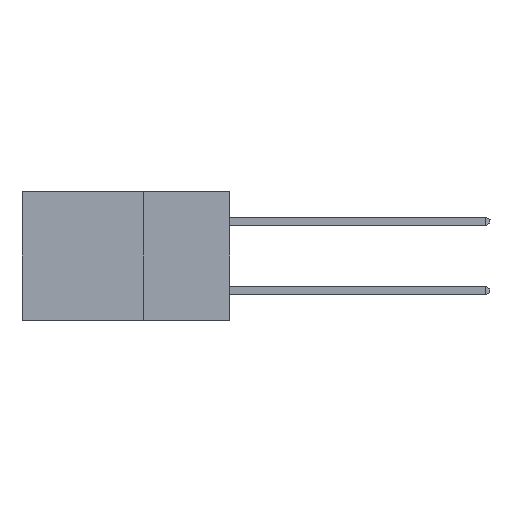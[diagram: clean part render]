
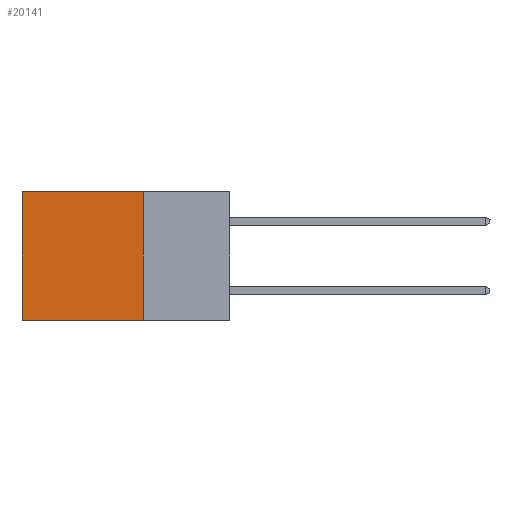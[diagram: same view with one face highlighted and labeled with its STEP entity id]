
A CAD part, left-side view. The second image highlights one B-rep face of the part: STEP entity #20141.
In plain terms, the highlighted planar face has unit normal (-1, 0, 0).
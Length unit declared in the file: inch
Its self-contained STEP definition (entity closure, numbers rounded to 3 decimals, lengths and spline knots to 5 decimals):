
#541 = VERTEX_POINT ( 'NONE', #21755 ) ;
#1035 = DIRECTION ( 'NONE',  ( 0., 0., -1. ) ) ;
#1156 = ORIENTED_EDGE ( 'NONE', *, *, #18524, .T. ) ;
#1758 = ORIENTED_EDGE ( 'NONE', *, *, #5226, .F. ) ;
#1939 = VERTEX_POINT ( 'NONE', #11589 ) ;
#2657 = VECTOR ( 'NONE', #6540, 39.37008 ) ;
#2949 = VECTOR ( 'NONE', #1035, 39.37008 ) ;
#4043 = EDGE_CURVE ( 'NONE', #1939, #17768, #13475, .T. ) ;
#4757 = CARTESIAN_POINT ( 'NONE',  ( 0.298, 0.25, -0.37 ) ) ;
#5226 = EDGE_CURVE ( 'NONE', #541, #17768, #16726, .T. ) ;
#6540 = DIRECTION ( 'NONE',  ( 0., 1., 0. ) ) ;
#6565 = CARTESIAN_POINT ( 'NONE',  ( 0.298, 0.25, 0. ) ) ;
#7012 = CARTESIAN_POINT ( 'NONE',  ( 0.298, 0.25, 0. ) ) ;
#9337 = VECTOR ( 'NONE', #22537, 39.37008 ) ;
#9915 = DIRECTION ( 'NONE',  ( 0., 0., -1. ) ) ;
#11246 = ORIENTED_EDGE ( 'NONE', *, *, #20131, .F. ) ;
#11589 = CARTESIAN_POINT ( 'NONE',  ( 0.298, 0.6, 0. ) ) ;
#12264 = VERTEX_POINT ( 'NONE', #7012 ) ;
#12310 = FACE_OUTER_BOUND ( 'NONE', #22610, .T. ) ;
#13475 = LINE ( 'NONE', #19010, #9337 ) ;
#16726 = LINE ( 'NONE', #4757, #2657 ) ;
#16926 = PLANE ( 'NONE',  #17272 ) ;
#17272 = AXIS2_PLACEMENT_3D ( 'NONE', #18714, #20440, #9915 ) ;
#17566 = LINE ( 'NONE', #22097, #2949 ) ;
#17768 = VERTEX_POINT ( 'NONE', #19486 ) ;
#18524 = EDGE_CURVE ( 'NONE', #12264, #1939, #18699, .T. ) ;
#18699 = LINE ( 'NONE', #6565, #22210 ) ;
#18714 = CARTESIAN_POINT ( 'NONE',  ( 0.298, 0.25, 0. ) ) ;
#19010 = CARTESIAN_POINT ( 'NONE',  ( 0.298, 0.6, 0. ) ) ;
#19486 = CARTESIAN_POINT ( 'NONE',  ( 0.298, 0.6, -0.37 ) ) ;
#20121 = ORIENTED_EDGE ( 'NONE', *, *, #4043, .T. ) ;
#20131 = EDGE_CURVE ( 'NONE', #12264, #541, #17566, .T. ) ;
#20141 = ADVANCED_FACE ( 'NONE', ( #12310 ), #16926, .F. ) ;
#20440 = DIRECTION ( 'NONE',  ( 1., 0., 0. ) ) ;
#20620 = DIRECTION ( 'NONE',  ( 0., 1., 0. ) ) ;
#21755 = CARTESIAN_POINT ( 'NONE',  ( 0.298, 0.25, -0.37 ) ) ;
#22097 = CARTESIAN_POINT ( 'NONE',  ( 0.298, 0.25, 0. ) ) ;
#22210 = VECTOR ( 'NONE', #20620, 39.37008 ) ;
#22537 = DIRECTION ( 'NONE',  ( 0., 0., -1. ) ) ;
#22610 = EDGE_LOOP ( 'NONE', ( #20121, #1758, #11246, #1156 ) ) ;
